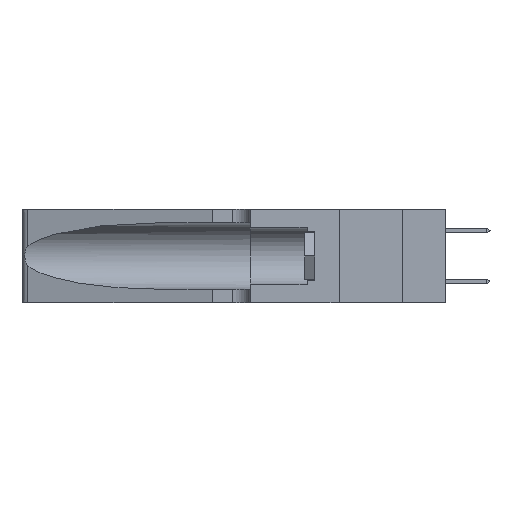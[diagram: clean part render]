
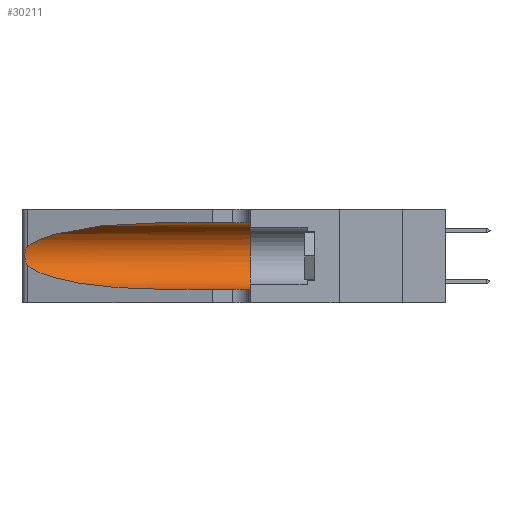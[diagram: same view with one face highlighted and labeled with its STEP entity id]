
A CAD part, left-side view. The second image highlights one B-rep face of the part: STEP entity #30211.
In plain terms, the highlighted cylindrical face has radius 3.308 mm (diameter 6.617 mm), a partial arc.
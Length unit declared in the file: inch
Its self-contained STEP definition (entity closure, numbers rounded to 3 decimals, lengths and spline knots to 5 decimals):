
#501 = ORIENTED_EDGE ( 'NONE', *, *, #11513, .T. ) ;
#632 = CARTESIAN_POINT ( 'NONE',  ( 0.25639, 1.23186, 0.15144 ) ) ;
#885 = CIRCLE ( 'NONE', #26122, 0.13025 ) ;
#1890 = CARTESIAN_POINT ( 'NONE',  ( 0.2373, 1.15595, 0.08982 ) ) ;
#2739 = LINE ( 'NONE', #24472, #20889 ) ;
#3927 = CARTESIAN_POINT ( 'NONE',  ( 0.25854, 1.2359, 0.20912 ) ) ;
#4403 = ORIENTED_EDGE ( 'NONE', *, *, #25223, .F. ) ;
#4601 = CARTESIAN_POINT ( 'NONE',  ( 0.25487, 1.22718, 0.22369 ) ) ;
#4719 = DIRECTION ( 'NONE',  ( 0., 1., 0. ) ) ;
#4758 = CARTESIAN_POINT ( 'NONE',  ( 0.1305, 0.72297, 0.31525 ) ) ;
#5285 = CARTESIAN_POINT ( 'NONE',  ( 0.1305, 0.35, 0.05475 ) ) ;
#5512 = CARTESIAN_POINT ( 'NONE',  ( 0.1305, 0.35, 0.31525 ) ) ;
#6406 = VECTOR ( 'NONE', #24525, 39.37008 ) ;
#6649 = CARTESIAN_POINT ( 'NONE',  ( 0.25555, 1.22994, 0.2215 ) ) ;
#7479 = EDGE_CURVE ( 'NONE', #8620, #26765, #32163, .T. ) ;
#8620 = VERTEX_POINT ( 'NONE', #24291 ) ;
#9400 = CARTESIAN_POINT ( 'NONE',  ( 0.25639, 1.23184, 0.21858 ) ) ;
#9734 = DIRECTION ( 'NONE',  ( 0., -1., 0. ) ) ;
#11513 = EDGE_CURVE ( 'NONE', #26623, #23256, #24246, .T. ) ;
#11868 = DIRECTION ( 'NONE',  ( 0., -1., 0. ) ) ;
#12124 = ORIENTED_EDGE ( 'NONE', *, *, #7479, .T. ) ;
#12260 = CARTESIAN_POINT ( 'NONE',  ( 0.25787, 1.23484, 0.2124 ) ) ;
#12388 = CARTESIAN_POINT ( 'NONE',  ( 0.25789, 1.23486, 0.15765 ) ) ;
#14906 = CARTESIAN_POINT ( 'NONE',  ( 0.25487, 1.22718, 0.14631 ) ) ;
#15227 = DIRECTION ( 'NONE',  ( 0., 0., -1. ) ) ;
#16981 = CARTESIAN_POINT ( 'NONE',  ( 0.1305, 0.72297, 0.05475 ) ) ;
#17085 = EDGE_CURVE ( 'NONE', #23256, #32871, #2739, .T. ) ;
#17521 = CARTESIAN_POINT ( 'NONE',  ( 0.25487, 1.22718, 0.14631 ) ) ;
#18430 = EDGE_LOOP ( 'NONE', ( #12124, #29956, #501, #27072, #4403, #30413 ) ) ;
#18503 = CARTESIAN_POINT ( 'NONE',  ( 0.26075, 1.23896, 0.178 ) ) ;
#18642 = CARTESIAN_POINT ( 'NONE',  ( 0.26017, 1.23833, 0.17102 ) ) ;
#19706 = AXIS2_PLACEMENT_3D ( 'NONE', #26747, #11868, #15227 ) ;
#20058 = FACE_OUTER_BOUND ( 'NONE', #18430, .T. ) ;
#20889 = VECTOR ( 'NONE', #9734, 39.37008 ) ;
#21793 = CARTESIAN_POINT ( 'NONE',  ( 0.25487, 1.22718, 0.22369 ) ) ;
#23256 = VERTEX_POINT ( 'NONE', #27719 ) ;
#23700 = CARTESIAN_POINT ( 'NONE',  ( 0.18966, 0.96281, 0.05475 ) ) ;
#24246 =( BOUNDED_CURVE ( )  B_SPLINE_CURVE ( 3, ( #14906, #1890, #23700, #16981 ),
 .UNSPECIFIED., .F., .F. ) 
 B_SPLINE_CURVE_WITH_KNOTS ( ( 4, 4 ),
 ( 3.44316, 4.71239 ),
 .UNSPECIFIED. ) 
 CURVE ( )  GEOMETRIC_REPRESENTATION_ITEM ( )  RATIONAL_B_SPLINE_CURVE ( ( 1., 0.87, 0.87, 1. ) ) 
 REPRESENTATION_ITEM ( '' )  );
#24291 = CARTESIAN_POINT ( 'NONE',  ( 0.1305, 0.72297, 0.31525 ) ) ;
#24472 = CARTESIAN_POINT ( 'NONE',  ( 0.1305, 1.61858, 0.05475 ) ) ;
#24525 = DIRECTION ( 'NONE',  ( 0., -1., 0. ) ) ;
#24666 = CARTESIAN_POINT ( 'NONE',  ( 0.25856, 1.23593, 0.16098 ) ) ;
#24792 = CARTESIAN_POINT ( 'NONE',  ( 0.26075, 1.23896, 0.19203 ) ) ;
#25223 = EDGE_CURVE ( 'NONE', #38430, #32871, #885, .T. ) ;
#25368 = CARTESIAN_POINT ( 'NONE',  ( 0.25487, 1.22718, 0.22369 ) ) ;
#26122 = AXIS2_PLACEMENT_3D ( 'NONE', #35017, #4719, #26126 ) ;
#26126 = DIRECTION ( 'NONE',  ( 0., 0., 1. ) ) ;
#26623 = VERTEX_POINT ( 'NONE', #17521 ) ;
#26747 = CARTESIAN_POINT ( 'NONE',  ( 0.1305, 1.61858, 0.185 ) ) ;
#26765 = VERTEX_POINT ( 'NONE', #4601 ) ;
#26877 = EDGE_CURVE ( 'NONE', #8620, #38430, #33050, .T. ) ;
#27072 = ORIENTED_EDGE ( 'NONE', *, *, #17085, .T. ) ;
#27509 = CYLINDRICAL_SURFACE ( 'NONE', #19706, 0.13025 ) ;
#27719 = CARTESIAN_POINT ( 'NONE',  ( 0.1305, 0.72297, 0.05475 ) ) ;
#29956 = ORIENTED_EDGE ( 'NONE', *, *, #31225, .T. ) ;
#30211 = ADVANCED_FACE ( 'NONE', ( #20058 ), #27509, .F. ) ;
#30413 = ORIENTED_EDGE ( 'NONE', *, *, #26877, .F. ) ;
#30697 = CARTESIAN_POINT ( 'NONE',  ( 0.25487, 1.22718, 0.14631 ) ) ;
#31225 = EDGE_CURVE ( 'NONE', #26765, #26623, #38146, .T. ) ;
#31405 = CARTESIAN_POINT ( 'NONE',  ( 0.2373, 1.15595, 0.28018 ) ) ;
#32163 =( BOUNDED_CURVE ( )  B_SPLINE_CURVE ( 3, ( #4758, #37219, #31405, #25368 ),
 .UNSPECIFIED., .F., .T. ) 
 B_SPLINE_CURVE_WITH_KNOTS ( ( 4, 4 ),
 ( 1.5708, 2.84003 ),
 .UNSPECIFIED. ) 
 CURVE ( )  GEOMETRIC_REPRESENTATION_ITEM ( )  RATIONAL_B_SPLINE_CURVE ( ( 1., 0.87, 0.87, 1. ) ) 
 REPRESENTATION_ITEM ( '' )  );
#32871 = VERTEX_POINT ( 'NONE', #5285 ) ;
#33050 = LINE ( 'NONE', #33812, #6406 ) ;
#33812 = CARTESIAN_POINT ( 'NONE',  ( 0.1305, 1.61858, 0.31525 ) ) ;
#35017 = CARTESIAN_POINT ( 'NONE',  ( 0.1305, 0.35, 0.185 ) ) ;
#36159 = CARTESIAN_POINT ( 'NONE',  ( 0.25555, 1.22993, 0.14849 ) ) ;
#36409 = CARTESIAN_POINT ( 'NONE',  ( 0.26018, 1.23835, 0.19895 ) ) ;
#37219 = CARTESIAN_POINT ( 'NONE',  ( 0.18966, 0.96281, 0.31525 ) ) ;
#38146 = B_SPLINE_CURVE_WITH_KNOTS ( 'NONE', 3,
 ( #21793, #6649, #9400, #12260, #3927, #36409, #24792, #18503, #18642, #24666, #12388, #632, #36159, #30697 ),
 .UNSPECIFIED., .F., .F.,
 ( 4, 2, 2, 2, 2, 2, 4 ),
 ( 0., 0.00027, 0.00053, 0.00107, 0.0016, 0.00187, 0.00214 ),
 .UNSPECIFIED. ) ;
#38430 = VERTEX_POINT ( 'NONE', #5512 ) ;
